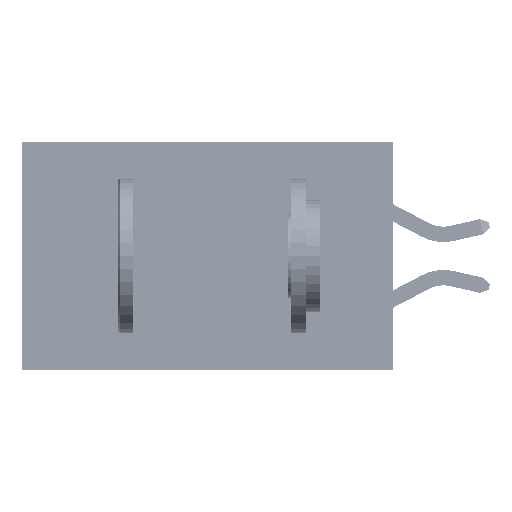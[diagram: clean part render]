
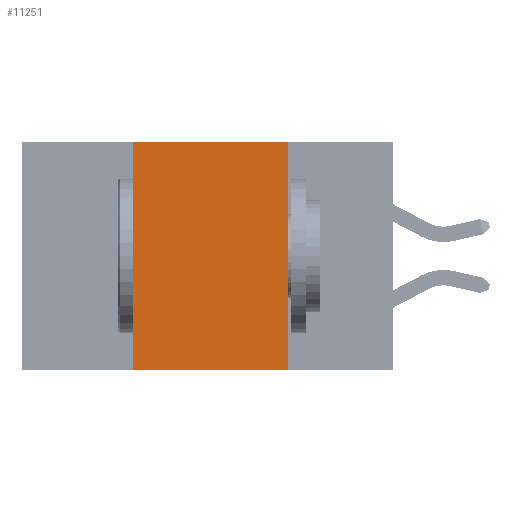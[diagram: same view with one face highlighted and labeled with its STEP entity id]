
A CAD part, left-side view. The second image highlights one B-rep face of the part: STEP entity #11251.
In plain terms, the highlighted planar face has unit normal (-1, 0, 0).
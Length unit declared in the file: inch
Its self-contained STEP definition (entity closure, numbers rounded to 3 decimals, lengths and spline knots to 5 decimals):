
#1442 = CARTESIAN_POINT ( 'NONE',  ( 0., 0.17, -0.37 ) ) ;
#2499 = LINE ( 'NONE', #8899, #49171 ) ;
#4230 = CARTESIAN_POINT ( 'NONE',  ( 0., 0.17, 0. ) ) ;
#6775 = CARTESIAN_POINT ( 'NONE',  ( 0., 0.6, -0.37 ) ) ;
#7743 = VECTOR ( 'NONE', #11232, 39.37008 ) ;
#8899 = CARTESIAN_POINT ( 'NONE',  ( 0., 0.6, 0. ) ) ;
#10608 = LINE ( 'NONE', #6775, #24900 ) ;
#11232 = DIRECTION ( 'NONE',  ( 0., 0., 1. ) ) ;
#11251 = ADVANCED_FACE ( 'NONE', ( #44466 ), #28470, .F. ) ;
#11483 = DIRECTION ( 'NONE',  ( 0., 0., -1. ) ) ;
#11669 = EDGE_CURVE ( 'NONE', #12695, #46046, #37611, .T. ) ;
#12695 = VERTEX_POINT ( 'NONE', #32277 ) ;
#13816 = EDGE_CURVE ( 'NONE', #50083, #18772, #24334, .T. ) ;
#18772 = VERTEX_POINT ( 'NONE', #1442 ) ;
#19015 = DIRECTION ( 'NONE',  ( 0., -1., 0. ) ) ;
#20253 = DIRECTION ( 'NONE',  ( 0., -1., 0. ) ) ;
#21230 = EDGE_CURVE ( 'NONE', #46046, #50083, #2499, .T. ) ;
#24127 = DIRECTION ( 'NONE',  ( 0., 0., -1. ) ) ;
#24334 = LINE ( 'NONE', #35659, #33660 ) ;
#24653 = DIRECTION ( 'NONE',  ( 1., 0., 0. ) ) ;
#24900 = VECTOR ( 'NONE', #19015, 39.37008 ) ;
#28421 = ORIENTED_EDGE ( 'NONE', *, *, #21230, .F. ) ;
#28470 = PLANE ( 'NONE',  #51177 ) ;
#30164 = EDGE_LOOP ( 'NONE', ( #49033, #28421, #38285, #35241 ) ) ;
#32277 = CARTESIAN_POINT ( 'NONE',  ( 0., 0.42, -0.37 ) ) ;
#33660 = VECTOR ( 'NONE', #11483, 39.37008 ) ;
#35241 = ORIENTED_EDGE ( 'NONE', *, *, #36060, .T. ) ;
#35539 = CARTESIAN_POINT ( 'NONE',  ( 0., 0.42, 0. ) ) ;
#35659 = CARTESIAN_POINT ( 'NONE',  ( 0., 0.17, 0. ) ) ;
#36060 = EDGE_CURVE ( 'NONE', #12695, #18772, #10608, .T. ) ;
#36838 = CARTESIAN_POINT ( 'NONE',  ( 0., 0.6, 0. ) ) ;
#37611 = LINE ( 'NONE', #50526, #7743 ) ;
#38285 = ORIENTED_EDGE ( 'NONE', *, *, #11669, .F. ) ;
#44466 = FACE_OUTER_BOUND ( 'NONE', #30164, .T. ) ;
#46046 = VERTEX_POINT ( 'NONE', #35539 ) ;
#49033 = ORIENTED_EDGE ( 'NONE', *, *, #13816, .F. ) ;
#49171 = VECTOR ( 'NONE', #20253, 39.37008 ) ;
#50083 = VERTEX_POINT ( 'NONE', #4230 ) ;
#50526 = CARTESIAN_POINT ( 'NONE',  ( 0., 0.42, 0. ) ) ;
#51177 = AXIS2_PLACEMENT_3D ( 'NONE', #36838, #24653, #24127 ) ;
